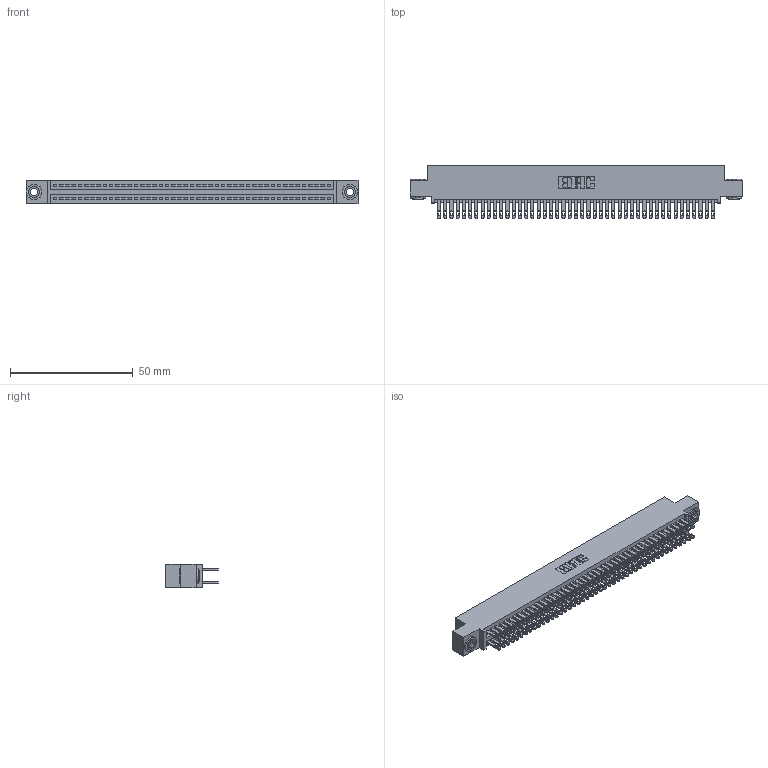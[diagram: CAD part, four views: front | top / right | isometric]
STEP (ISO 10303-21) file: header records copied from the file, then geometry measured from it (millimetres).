
FILE_DESCRIPTION (( 'STEP AP203' ), '1' );
FILE_NAME ('345-090-500-503.STEP', '2018-10-04T15:42:07', ( '' ), ( '' ), 'SwSTEP 2.0', 'SolidWorks 2016', '' );
FILE_SCHEMA (( 'CONFIG_CONTROL_DESIGN' ));
Length unit declared in the file: inch
Products named in the file (4): 345-250-002_345-250-002-102; 345 Part_0.110 Offset - 0.156 Dia-TH; 345-292-001_345-293-100; 345-090-500-503
Assembly tree (93 placements, depth 2):
  345-090-500-503
    345 Part_0.110 Offset - 0.156 Dia-TH
    345-292-001_345-293-100  x90
    345-250-002_345-250-002-102  x2
Bounding box: 135.51 x 21.51 x 9.4 mm (x, y, z)
Volume: 13412.4 mm3; surface area: 21099.5 mm2
Topology: 93 solids, 93 shells, 4308 faces, 13119 edges, 8742 vertices
Faces by surface type: plane 2524, cylinder 1776, cone 8
Entity records: 35616 total; most frequent: CARTESIAN_POINT 5943, ORIENTED_EDGE 5870, DIRECTION 5269, EDGE_CURVE 2935, VECTOR 2595, LINE 2595, VERTEX_POINT 1954, AXIS2_PLACEMENT_3D 1337
